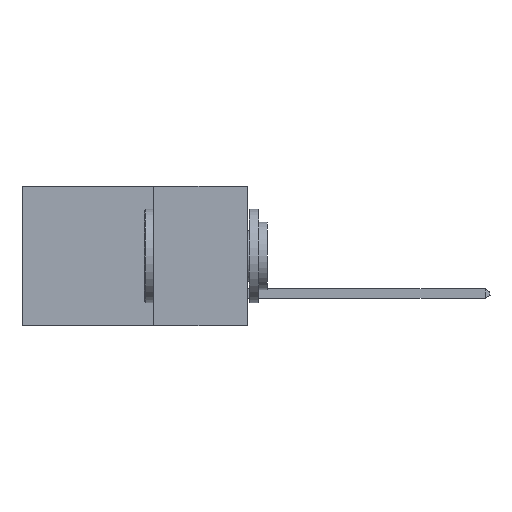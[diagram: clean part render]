
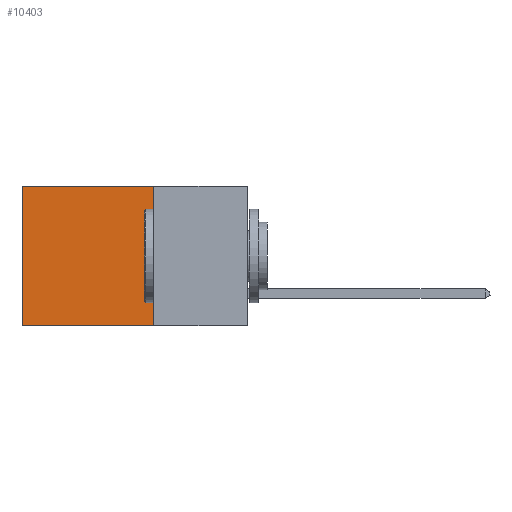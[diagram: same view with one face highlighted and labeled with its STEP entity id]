
A CAD part, left-side view. The second image highlights one B-rep face of the part: STEP entity #10403.
In plain terms, the highlighted planar face has unit normal (-1, 0, 0).
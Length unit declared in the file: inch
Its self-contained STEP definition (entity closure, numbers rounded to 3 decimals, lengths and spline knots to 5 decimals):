
#231 = DIRECTION ( 'NONE',  ( 0., 0., -1. ) ) ;
#701 = CARTESIAN_POINT ( 'NONE',  ( 0.298, 0.6, -0.37 ) ) ;
#1138 = LINE ( 'NONE', #8787, #10073 ) ;
#2336 = ORIENTED_EDGE ( 'NONE', *, *, #5574, .T. ) ;
#3281 = ORIENTED_EDGE ( 'NONE', *, *, #10324, .F. ) ;
#3307 = CARTESIAN_POINT ( 'NONE',  ( 0.298, 0.25, 0. ) ) ;
#3313 = DIRECTION ( 'NONE',  ( 1., 0., 0. ) ) ;
#3859 = AXIS2_PLACEMENT_3D ( 'NONE', #9278, #3313, #4191 ) ;
#4191 = DIRECTION ( 'NONE',  ( 0., 0., -1. ) ) ;
#4275 = VECTOR ( 'NONE', #6059, 39.37008 ) ;
#4434 = ORIENTED_EDGE ( 'NONE', *, *, #8422, .F. ) ;
#4673 = VERTEX_POINT ( 'NONE', #4742 ) ;
#4742 = CARTESIAN_POINT ( 'NONE',  ( 0.298, 0.25, -0.37 ) ) ;
#4817 = LINE ( 'NONE', #3307, #4275 ) ;
#4927 = VERTEX_POINT ( 'NONE', #701 ) ;
#5260 = DIRECTION ( 'NONE',  ( 0., 1., 0. ) ) ;
#5422 = CARTESIAN_POINT ( 'NONE',  ( 0.298, 0.6, 0. ) ) ;
#5574 = EDGE_CURVE ( 'NONE', #7997, #4927, #10334, .T. ) ;
#6011 = LINE ( 'NONE', #9534, #9773 ) ;
#6059 = DIRECTION ( 'NONE',  ( 0., 1., 0. ) ) ;
#7526 = PLANE ( 'NONE',  #3859 ) ;
#7997 = VERTEX_POINT ( 'NONE', #8896 ) ;
#8173 = DIRECTION ( 'NONE',  ( 0., 0., -1. ) ) ;
#8422 = EDGE_CURVE ( 'NONE', #4673, #4927, #6011, .T. ) ;
#8512 = EDGE_CURVE ( 'NONE', #10340, #7997, #4817, .T. ) ;
#8787 = CARTESIAN_POINT ( 'NONE',  ( 0.298, 0.25, 0. ) ) ;
#8896 = CARTESIAN_POINT ( 'NONE',  ( 0.298, 0.6, 0. ) ) ;
#9278 = CARTESIAN_POINT ( 'NONE',  ( 0.298, 0.25, 0. ) ) ;
#9316 = VECTOR ( 'NONE', #231, 39.37008 ) ;
#9446 = FACE_OUTER_BOUND ( 'NONE', #9658, .T. ) ;
#9534 = CARTESIAN_POINT ( 'NONE',  ( 0.298, 0.25, -0.37 ) ) ;
#9658 = EDGE_LOOP ( 'NONE', ( #2336, #4434, #3281, #10322 ) ) ;
#9773 = VECTOR ( 'NONE', #5260, 39.37008 ) ;
#9957 = CARTESIAN_POINT ( 'NONE',  ( 0.298, 0.25, 0. ) ) ;
#10073 = VECTOR ( 'NONE', #8173, 39.37008 ) ;
#10322 = ORIENTED_EDGE ( 'NONE', *, *, #8512, .T. ) ;
#10324 = EDGE_CURVE ( 'NONE', #10340, #4673, #1138, .T. ) ;
#10334 = LINE ( 'NONE', #5422, #9316 ) ;
#10340 = VERTEX_POINT ( 'NONE', #9957 ) ;
#10403 = ADVANCED_FACE ( 'NONE', ( #9446 ), #7526, .F. ) ;
